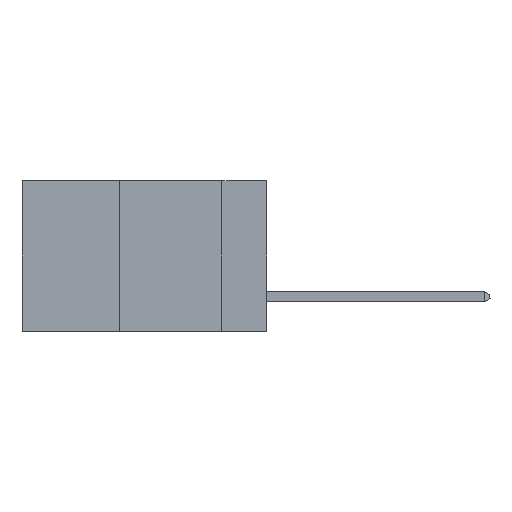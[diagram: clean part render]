
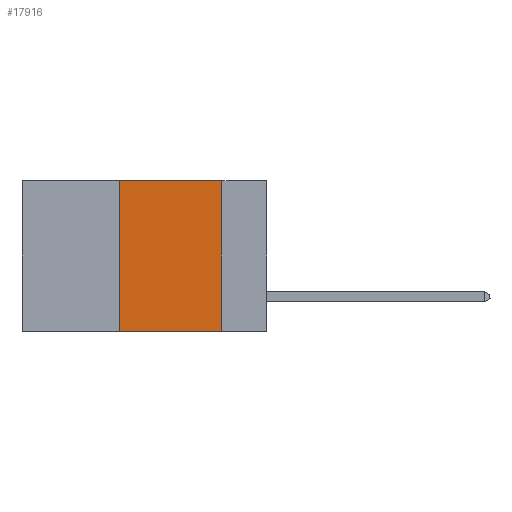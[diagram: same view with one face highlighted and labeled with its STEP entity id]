
A CAD part, left-side view. The second image highlights one B-rep face of the part: STEP entity #17916.
In plain terms, the highlighted planar face has unit normal (-1, 0, 0).
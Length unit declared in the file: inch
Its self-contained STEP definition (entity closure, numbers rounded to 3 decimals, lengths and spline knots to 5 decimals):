
#40 = EDGE_CURVE ( 'NONE', #4684, #11851, #3456, .T. ) ;
#706 = CARTESIAN_POINT ( 'NONE',  ( 0., 0.6, 0. ) ) ;
#3373 = CARTESIAN_POINT ( 'NONE',  ( 0., 0.6, -0.37 ) ) ;
#3456 = LINE ( 'NONE', #10728, #10914 ) ;
#3784 = EDGE_CURVE ( 'NONE', #17539, #12056, #4514, .T. ) ;
#3820 = EDGE_CURVE ( 'NONE', #17539, #4684, #7966, .T. ) ;
#4514 = LINE ( 'NONE', #3373, #12006 ) ;
#4684 = VERTEX_POINT ( 'NONE', #9820 ) ;
#4826 = ORIENTED_EDGE ( 'NONE', *, *, #3784, .T. ) ;
#4925 = DIRECTION ( 'NONE',  ( 0., 0., 1. ) ) ;
#5634 = CARTESIAN_POINT ( 'NONE',  ( 0., 0.11, -0.37 ) ) ;
#6681 = PLANE ( 'NONE',  #13608 ) ;
#7891 = DIRECTION ( 'NONE',  ( 0., 0., -1. ) ) ;
#7966 = LINE ( 'NONE', #10931, #15988 ) ;
#8196 = DIRECTION ( 'NONE',  ( 0., 0., -1. ) ) ;
#8818 = EDGE_CURVE ( 'NONE', #11851, #12056, #15344, .T. ) ;
#9820 = CARTESIAN_POINT ( 'NONE',  ( 0., 0.36, 0. ) ) ;
#10728 = CARTESIAN_POINT ( 'NONE',  ( 0., 0.6, 0. ) ) ;
#10914 = VECTOR ( 'NONE', #13840, 39.37008 ) ;
#10931 = CARTESIAN_POINT ( 'NONE',  ( 0., 0.36, 0. ) ) ;
#11164 = CARTESIAN_POINT ( 'NONE',  ( 0., 0.11, 0. ) ) ;
#11281 = EDGE_LOOP ( 'NONE', ( #14909, #15370, #19273, #4826 ) ) ;
#11325 = FACE_OUTER_BOUND ( 'NONE', #11281, .T. ) ;
#11816 = VECTOR ( 'NONE', #7891, 39.37008 ) ;
#11851 = VERTEX_POINT ( 'NONE', #11164 ) ;
#12006 = VECTOR ( 'NONE', #12399, 39.37008 ) ;
#12056 = VERTEX_POINT ( 'NONE', #5634 ) ;
#12399 = DIRECTION ( 'NONE',  ( 0., -1., 0. ) ) ;
#13608 = AXIS2_PLACEMENT_3D ( 'NONE', #706, #17248, #8196 ) ;
#13840 = DIRECTION ( 'NONE',  ( 0., -1., 0. ) ) ;
#13951 = CARTESIAN_POINT ( 'NONE',  ( 0., 0.11, 0. ) ) ;
#14909 = ORIENTED_EDGE ( 'NONE', *, *, #8818, .F. ) ;
#15344 = LINE ( 'NONE', #13951, #11816 ) ;
#15370 = ORIENTED_EDGE ( 'NONE', *, *, #40, .F. ) ;
#15988 = VECTOR ( 'NONE', #4925, 39.37008 ) ;
#17248 = DIRECTION ( 'NONE',  ( 1., 0., 0. ) ) ;
#17539 = VERTEX_POINT ( 'NONE', #18955 ) ;
#17916 = ADVANCED_FACE ( 'NONE', ( #11325 ), #6681, .F. ) ;
#18955 = CARTESIAN_POINT ( 'NONE',  ( 0., 0.36, -0.37 ) ) ;
#19273 = ORIENTED_EDGE ( 'NONE', *, *, #3820, .F. ) ;
